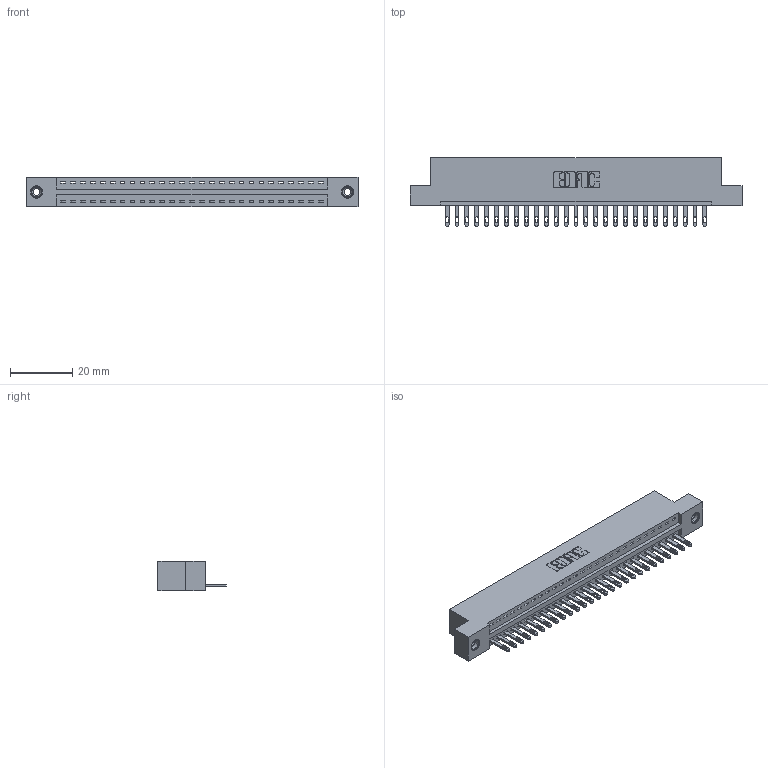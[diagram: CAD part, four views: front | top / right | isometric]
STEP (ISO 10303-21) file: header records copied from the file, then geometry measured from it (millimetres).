
FILE_DESCRIPTION (( 'STEP AP203' ), '1' );
FILE_NAME ('896-027-500-108.STEP', '2021-07-27T18:07:45', ( '' ), ( '' ), 'SwSTEP 2.0', 'SolidWorks 2020', '' );
FILE_SCHEMA (( 'CONFIG_CONTROL_DESIGN' ));
Length unit declared in the file: inch
Products named in the file (4): 345-250-001_345-250-003-102; 896-027-500-108; 846 Part_Flush Mounting Lugs - 0.156 Dia-TI; 345-292-001_345-293-100
Assembly tree (30 placements, depth 2):
  896-027-500-108
    846 Part_Flush Mounting Lugs - 0.156 Dia-TI
    345-292-001_345-293-100  x27
    345-250-001_345-250-003-102  x2
Bounding box: 106.3 x 21.84 x 9.4 mm (x, y, z)
Volume: 10082 mm3; surface area: 12524.1 mm2
Topology: 30 solids, 30 shells, 1640 faces, 5001 edges, 3326 vertices
Faces by surface type: plane 1026, cylinder 598, cone 12, torus 4
Entity records: 19892 total; most frequent: CARTESIAN_POINT 3396, ORIENTED_EDGE 3350, DIRECTION 3043, EDGE_CURVE 1675, LINE 1411, VECTOR 1411, VERTEX_POINT 1112, AXIS2_PLACEMENT_3D 816
